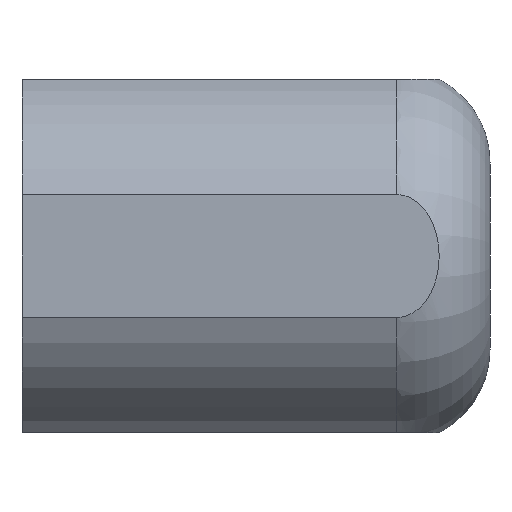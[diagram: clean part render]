
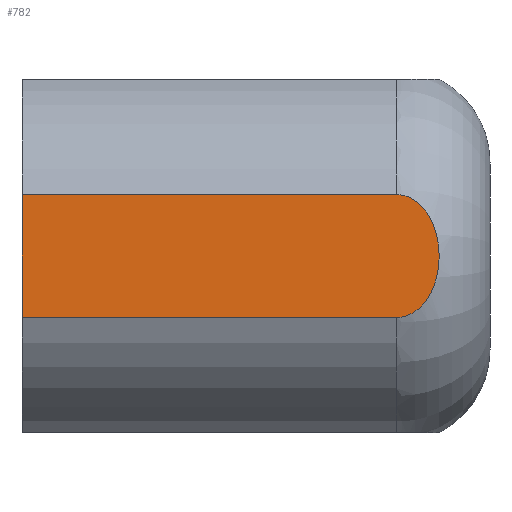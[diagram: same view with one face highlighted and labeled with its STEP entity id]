
A CAD part, left-side view. The second image highlights one B-rep face of the part: STEP entity #782.
In plain terms, the highlighted planar face has unit normal (-1, 0, 0).
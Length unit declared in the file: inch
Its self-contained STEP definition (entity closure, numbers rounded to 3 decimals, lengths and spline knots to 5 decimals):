
#9 = B_SPLINE_CURVE_WITH_KNOTS ( 'NONE', 3,
 ( #103, #106, #116, #110, #108, #111, #94, #95, #119, #112, #145, #147, #137, #146, #127, #154, #148, #129, #139, #152, #130, #143, #133, #149, #156, #138, #132, #150, #144, #131, #128, #134, #151, #125, #155, #135 ),
 .UNSPECIFIED., .F., .F.,
 ( 4, 2, 2, 2, 2, 2, 2, 2, 2, 2, 2, 2, 2, 2, 2, 2, 2, 4 ),
 ( 0., 0.00084, 0.00126, 0.00168, 0.0021, 0.00252, 0.00336, 0.00503, 0.00671, 0.00755, 0.00839, 0.00923, 0.01007, 0.01091, 0.01174, 0.01258, 0.013, 0.01342 ),
 .UNSPECIFIED. ) ;
#26 = DIRECTION ( 'NONE',  ( 0., 0., 1. ) ) ;
#28 = PLANE ( 'NONE',  #957 ) ;
#31 = DIRECTION ( 'NONE',  ( -1., 0., 0. ) ) ;
#35 = CARTESIAN_POINT ( 'NONE',  ( 0., 1.5, 0. ) ) ;
#94 = CARTESIAN_POINT ( 'NONE',  ( 0., 0.24249, -0.3762 ) ) ;
#95 = CARTESIAN_POINT ( 'NONE',  ( 0., 0.23346, -0.36977 ) ) ;
#103 = CARTESIAN_POINT ( 'NONE',  ( 0., 0.3, -0.3937 ) ) ;
#106 = CARTESIAN_POINT ( 'NONE',  ( 0., 0.28879, -0.3937 ) ) ;
#108 = CARTESIAN_POINT ( 'NONE',  ( 0., 0.25701, -0.38421 ) ) ;
#110 = CARTESIAN_POINT ( 'NONE',  ( 0., 0.26216, -0.38644 ) ) ;
#111 = CARTESIAN_POINT ( 'NONE',  ( 0., 0.2472, -0.3791 ) ) ;
#112 = CARTESIAN_POINT ( 'NONE',  ( 0., 0.22095, -0.35872 ) ) ;
#116 = CARTESIAN_POINT ( 'NONE',  ( 0., 0.27795, -0.39182 ) ) ;
#119 = CARTESIAN_POINT ( 'NONE',  ( 0., 0.22911, -0.36622 ) ) ;
#125 = CARTESIAN_POINT ( 'NONE',  ( 0., 0.28887, -0.00047 ) ) ;
#127 = CARTESIAN_POINT ( 'NONE',  ( 0., 0.17547, -0.28382 ) ) ;
#128 = CARTESIAN_POINT ( 'NONE',  ( 0., 0.25684, -0.00909 ) ) ;
#129 = CARTESIAN_POINT ( 'NONE',  ( 0., 0.16272, -0.18595 ) ) ;
#130 = CARTESIAN_POINT ( 'NONE',  ( 0., 0.16776, -0.14209 ) ) ;
#131 = CARTESIAN_POINT ( 'NONE',  ( 0., 0.24683, -0.0144 ) ) ;
#132 = CARTESIAN_POINT ( 'NONE',  ( 0., 0.2061, -0.05162 ) ) ;
#133 = CARTESIAN_POINT ( 'NONE',  ( 0., 0.17604, -0.1104 ) ) ;
#134 = CARTESIAN_POINT ( 'NONE',  ( 0., 0.27253, -0.00372 ) ) ;
#135 = CARTESIAN_POINT ( 'NONE',  ( 0., 0.3, 0. ) ) ;
#137 = CARTESIAN_POINT ( 'NONE',  ( 0., 0.19987, -0.33317 ) ) ;
#138 = CARTESIAN_POINT ( 'NONE',  ( 0., 0.19978, -0.06066 ) ) ;
#139 = CARTESIAN_POINT ( 'NONE',  ( 0., 0.16334, -0.17488 ) ) ;
#143 = CARTESIAN_POINT ( 'NONE',  ( 0., 0.17284, -0.12084 ) ) ;
#144 = CARTESIAN_POINT ( 'NONE',  ( 0., 0.22886, -0.02722 ) ) ;
#145 = CARTESIAN_POINT ( 'NONE',  ( 0., 0.21712, -0.35476 ) ) ;
#146 = CARTESIAN_POINT ( 'NONE',  ( 0., 0.18318, -0.30442 ) ) ;
#147 = CARTESIAN_POINT ( 'NONE',  ( 0., 0.20628, -0.34231 ) ) ;
#148 = CARTESIAN_POINT ( 'NONE',  ( 0., 0.16273, -0.21886 ) ) ;
#149 = CARTESIAN_POINT ( 'NONE',  ( 0., 0.18392, -0.08995 ) ) ;
#150 = CARTESIAN_POINT ( 'NONE',  ( 0., 0.22063, -0.03488 ) ) ;
#151 = CARTESIAN_POINT ( 'NONE',  ( 0., 0.27789, -0.00234 ) ) ;
#152 = CARTESIAN_POINT ( 'NONE',  ( 0., 0.16587, -0.1529 ) ) ;
#154 = CARTESIAN_POINT ( 'NONE',  ( 0., 0.16513, -0.24064 ) ) ;
#155 = CARTESIAN_POINT ( 'NONE',  ( 0., 0.29447, 0. ) ) ;
#156 = CARTESIAN_POINT ( 'NONE',  ( 0., 0.18866, -0.07985 ) ) ;
#226 = CARTESIAN_POINT ( 'NONE',  ( 0., 1.5, -0.3937 ) ) ;
#240 = DIRECTION ( 'NONE',  ( 0., -1., 0. ) ) ;
#242 = LINE ( 'NONE', #226, #860 ) ;
#260 = DIRECTION ( 'NONE',  ( 0., 0., -1. ) ) ;
#275 = CARTESIAN_POINT ( 'NONE',  ( 0., 1.5, 0. ) ) ;
#281 = LINE ( 'NONE', #275, #879 ) ;
#291 = DIRECTION ( 'NONE',  ( 0., -1., 0. ) ) ;
#301 = LINE ( 'NONE', #314, #901 ) ;
#314 = CARTESIAN_POINT ( 'NONE',  ( 0., 1.5, 0. ) ) ;
#455 = ORIENTED_EDGE ( 'NONE', *, *, #719, .T. ) ;
#460 = ORIENTED_EDGE ( 'NONE', *, *, #756, .F. ) ;
#471 = ORIENTED_EDGE ( 'NONE', *, *, #737, .T. ) ;
#476 = ORIENTED_EDGE ( 'NONE', *, *, #746, .T. ) ;
#485 = VERTEX_POINT ( 'NONE', #572 ) ;
#519 = EDGE_LOOP ( 'NONE', ( #471, #455, #460, #476 ) ) ;
#525 = VERTEX_POINT ( 'NONE', #582 ) ;
#531 = VERTEX_POINT ( 'NONE', #586 ) ;
#538 = VERTEX_POINT ( 'NONE', #603 ) ;
#572 = CARTESIAN_POINT ( 'NONE',  ( 0., 1.5, 0. ) ) ;
#582 = CARTESIAN_POINT ( 'NONE',  ( 0., 1.5, -0.3937 ) ) ;
#586 = CARTESIAN_POINT ( 'NONE',  ( 0., 0.3, 0. ) ) ;
#603 = CARTESIAN_POINT ( 'NONE',  ( 0., 0.3, -0.3937 ) ) ;
#719 = EDGE_CURVE ( 'NONE', #538, #531, #9, .T. ) ;
#737 = EDGE_CURVE ( 'NONE', #525, #538, #242, .T. ) ;
#746 = EDGE_CURVE ( 'NONE', #485, #525, #281, .T. ) ;
#756 = EDGE_CURVE ( 'NONE', #485, #531, #301, .T. ) ;
#782 = ADVANCED_FACE ( 'NONE', ( #945 ), #28, .T. ) ;
#860 = VECTOR ( 'NONE', #240, 39.37008 ) ;
#879 = VECTOR ( 'NONE', #260, 39.37008 ) ;
#901 = VECTOR ( 'NONE', #291, 39.37008 ) ;
#945 = FACE_OUTER_BOUND ( 'NONE', #519, .T. ) ;
#957 = AXIS2_PLACEMENT_3D ( 'NONE', #35, #31, #26 ) ;
